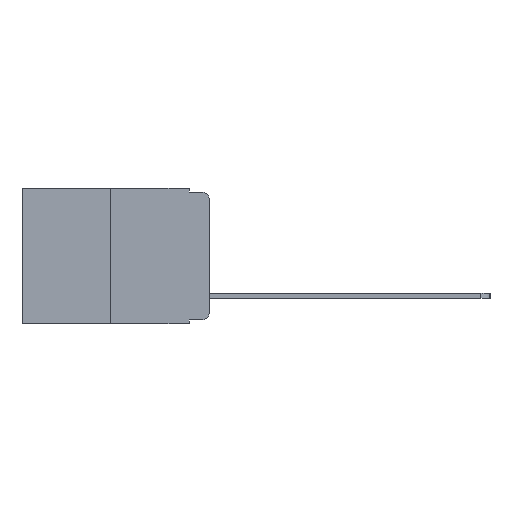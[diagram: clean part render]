
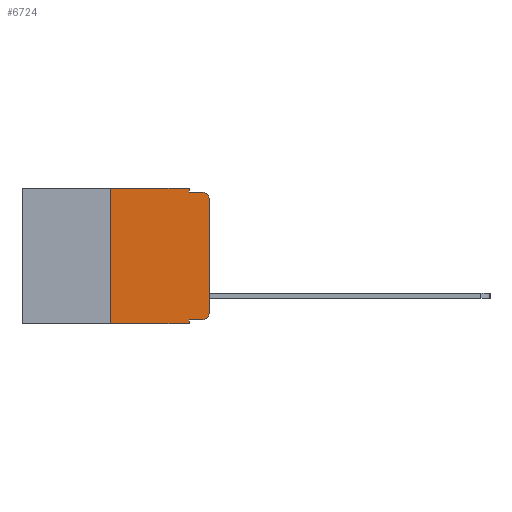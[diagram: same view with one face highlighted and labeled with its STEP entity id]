
A CAD part, left-side view. The second image highlights one B-rep face of the part: STEP entity #6724.
In plain terms, the highlighted planar face has unit normal (-1, 0, 0).
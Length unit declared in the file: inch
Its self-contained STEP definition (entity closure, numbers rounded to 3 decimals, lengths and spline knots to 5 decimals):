
#53 = EDGE_CURVE ( 'NONE', #1305, #6830, #11383, .T. ) ;
#389 = DIRECTION ( 'NONE',  ( 0., -1., 0. ) ) ;
#401 = DIRECTION ( 'NONE',  ( 0., 0., -1. ) ) ;
#1133 = ORIENTED_EDGE ( 'NONE', *, *, #4929, .F. ) ;
#1162 = DIRECTION ( 'NONE',  ( 0., 0., 1. ) ) ;
#1305 = VERTEX_POINT ( 'NONE', #14040 ) ;
#1347 = ORIENTED_EDGE ( 'NONE', *, *, #20181, .T. ) ;
#1471 = ORIENTED_EDGE ( 'NONE', *, *, #21264, .F. ) ;
#1476 = ORIENTED_EDGE ( 'NONE', *, *, #1645, .T. ) ;
#1574 = ORIENTED_EDGE ( 'NONE', *, *, #11374, .F. ) ;
#1645 = EDGE_CURVE ( 'NONE', #1305, #11653, #21137, .T. ) ;
#1672 = ORIENTED_EDGE ( 'NONE', *, *, #16942, .T. ) ;
#1746 = ORIENTED_EDGE ( 'NONE', *, *, #53, .F. ) ;
#1812 = ORIENTED_EDGE ( 'NONE', *, *, #2545, .F. ) ;
#1930 = ORIENTED_EDGE ( 'NONE', *, *, #6139, .T. ) ;
#1984 = DIRECTION ( 'NONE',  ( 0., 0., -1. ) ) ;
#2163 = ORIENTED_EDGE ( 'NONE', *, *, #9778, .T. ) ;
#2394 = VERTEX_POINT ( 'NONE', #13768 ) ;
#2415 = DIRECTION ( 'NONE',  ( 0., -1., 0. ) ) ;
#2545 = EDGE_CURVE ( 'NONE', #2394, #12329, #7014, .T. ) ;
#2576 = CARTESIAN_POINT ( 'NONE',  ( 0., 0.25, 0. ) ) ;
#3310 = DIRECTION ( 'NONE',  ( -1., 0., 0. ) ) ;
#4929 = EDGE_CURVE ( 'NONE', #12329, #19831, #8017, .T. ) ;
#5332 = LINE ( 'NONE', #11154, #7044 ) ;
#5712 = DIRECTION ( 'NONE',  ( 0., -1., 0. ) ) ;
#5781 = DIRECTION ( 'NONE',  ( -1., 0., 0. ) ) ;
#5921 = CARTESIAN_POINT ( 'NONE',  ( 0., 0.051, -0.01 ) ) ;
#6139 = EDGE_CURVE ( 'NONE', #12622, #19831, #21270, .T. ) ;
#6724 = ADVANCED_FACE ( 'NONE', ( #17721 ), #21036, .F. ) ;
#6830 = VERTEX_POINT ( 'NONE', #19557 ) ;
#7014 = LINE ( 'NONE', #14241, #7576 ) ;
#7044 = VECTOR ( 'NONE', #389, 39.37008 ) ;
#7576 = VECTOR ( 'NONE', #1984, 39.37008 ) ;
#8017 = LINE ( 'NONE', #5921, #20836 ) ;
#8926 = VERTEX_POINT ( 'NONE', #21462 ) ;
#9778 = EDGE_CURVE ( 'NONE', #8926, #12622, #14056, .T. ) ;
#9789 = CARTESIAN_POINT ( 'NONE',  ( 0., 0., 0. ) ) ;
#10109 = AXIS2_PLACEMENT_3D ( 'NONE', #16137, #5781, #17787 ) ;
#10675 = DIRECTION ( 'NONE',  ( 0., 0., -1. ) ) ;
#10989 = CARTESIAN_POINT ( 'NONE',  ( 0., 0.051, -0.333 ) ) ;
#11154 = CARTESIAN_POINT ( 'NONE',  ( 0., 0.051, -0.333 ) ) ;
#11168 = DIRECTION ( 'NONE',  ( 1., 0., 0. ) ) ;
#11253 = CARTESIAN_POINT ( 'NONE',  ( 0., 0., -0.03 ) ) ;
#11374 = EDGE_CURVE ( 'NONE', #6830, #2394, #15632, .T. ) ;
#11383 = LINE ( 'NONE', #2576, #19658 ) ;
#11487 = DIRECTION ( 'NONE',  ( 0., 0., 1. ) ) ;
#11653 = VERTEX_POINT ( 'NONE', #13414 ) ;
#12329 = VERTEX_POINT ( 'NONE', #15463 ) ;
#12622 = VERTEX_POINT ( 'NONE', #11253 ) ;
#12757 = DIRECTION ( 'NONE',  ( 0., -1., 0. ) ) ;
#13307 = CARTESIAN_POINT ( 'NONE',  ( 0., 0.02, -0.333 ) ) ;
#13414 = CARTESIAN_POINT ( 'NONE',  ( 0., 0.051, -0.343 ) ) ;
#13768 = CARTESIAN_POINT ( 'NONE',  ( 0., 0.051, 0. ) ) ;
#13827 = CARTESIAN_POINT ( 'NONE',  ( 0., 0.02, -0.03 ) ) ;
#14040 = CARTESIAN_POINT ( 'NONE',  ( 0., 0.25, -0.343 ) ) ;
#14056 = LINE ( 'NONE', #9789, #22231 ) ;
#14241 = CARTESIAN_POINT ( 'NONE',  ( 0., 0.051, 0. ) ) ;
#14469 = CARTESIAN_POINT ( 'NONE',  ( 0., 0.473, 0. ) ) ;
#15463 = CARTESIAN_POINT ( 'NONE',  ( 0., 0.051, -0.01 ) ) ;
#15550 = DIRECTION ( 'NONE',  ( 0., 0., -1. ) ) ;
#15632 = LINE ( 'NONE', #20896, #18443 ) ;
#15714 = CIRCLE ( 'NONE', #10109, 0.02 ) ;
#15839 = VECTOR ( 'NONE', #10675, 39.37008 ) ;
#15875 = AXIS2_PLACEMENT_3D ( 'NONE', #14469, #11168, #401 ) ;
#16009 = AXIS2_PLACEMENT_3D ( 'NONE', #13827, #3310, #15550 ) ;
#16137 = CARTESIAN_POINT ( 'NONE',  ( 0., 0.02, -0.313 ) ) ;
#16942 = EDGE_CURVE ( 'NONE', #19044, #8926, #15714, .T. ) ;
#17721 = FACE_OUTER_BOUND ( 'NONE', #20485, .T. ) ;
#17787 = DIRECTION ( 'NONE',  ( 0., 0., -1. ) ) ;
#18443 = VECTOR ( 'NONE', #5712, 39.37008 ) ;
#18803 = VERTEX_POINT ( 'NONE', #10989 ) ;
#18967 = CARTESIAN_POINT ( 'NONE',  ( 0., 0.051, 0. ) ) ;
#19044 = VERTEX_POINT ( 'NONE', #13307 ) ;
#19557 = CARTESIAN_POINT ( 'NONE',  ( 0., 0.25, 0. ) ) ;
#19658 = VECTOR ( 'NONE', #1162, 39.37008 ) ;
#19831 = VERTEX_POINT ( 'NONE', #20262 ) ;
#20144 = LINE ( 'NONE', #18967, #15839 ) ;
#20181 = EDGE_CURVE ( 'NONE', #18803, #19044, #5332, .T. ) ;
#20262 = CARTESIAN_POINT ( 'NONE',  ( 0., 0.02, -0.01 ) ) ;
#20485 = EDGE_LOOP ( 'NONE', ( #2163, #1930, #1133, #1812, #1574, #1746, #1476, #1471, #1347, #1672 ) ) ;
#20636 = VECTOR ( 'NONE', #12757, 39.37008 ) ;
#20836 = VECTOR ( 'NONE', #2415, 39.37008 ) ;
#20896 = CARTESIAN_POINT ( 'NONE',  ( 0., 0.473, 0. ) ) ;
#21036 = PLANE ( 'NONE',  #15875 ) ;
#21137 = LINE ( 'NONE', #21597, #20636 ) ;
#21264 = EDGE_CURVE ( 'NONE', #18803, #11653, #20144, .T. ) ;
#21270 = CIRCLE ( 'NONE', #16009, 0.02 ) ;
#21462 = CARTESIAN_POINT ( 'NONE',  ( 0., 0., -0.313 ) ) ;
#21597 = CARTESIAN_POINT ( 'NONE',  ( 0., 0.473, -0.343 ) ) ;
#22231 = VECTOR ( 'NONE', #11487, 39.37008 ) ;
